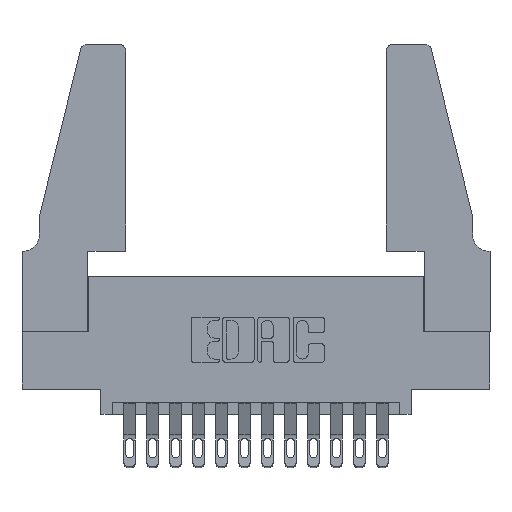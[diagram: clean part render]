
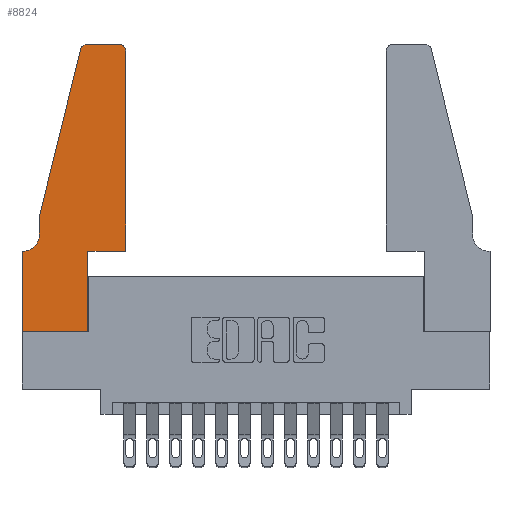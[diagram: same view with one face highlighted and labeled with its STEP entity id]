
A CAD part, top view. The second image highlights one B-rep face of the part: STEP entity #8824.
In plain terms, the highlighted planar face has unit normal (0, 0, 1).
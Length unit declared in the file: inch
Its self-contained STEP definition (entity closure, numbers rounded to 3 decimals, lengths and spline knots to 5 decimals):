
#144 = PLANE ( 'NONE',  #15446 ) ;
#333 = CARTESIAN_POINT ( 'NONE',  ( 0., 0.35, 0.37 ) ) ;
#470 = EDGE_CURVE ( 'NONE', #14573, #10132, #8382, .T. ) ;
#516 = ORIENTED_EDGE ( 'NONE', *, *, #2509, .T. ) ;
#527 = VECTOR ( 'NONE', #4725, 39.37008 ) ;
#585 = DIRECTION ( 'NONE',  ( 1., 0., 0. ) ) ;
#693 = CARTESIAN_POINT ( 'NONE',  ( 0.4205, 1.22, 0.37 ) ) ;
#936 = CARTESIAN_POINT ( 'NONE',  ( 0.0755, 0.35, 0.37 ) ) ;
#961 = EDGE_CURVE ( 'NONE', #8981, #6035, #6243, .T. ) ;
#1229 = ORIENTED_EDGE ( 'NONE', *, *, #961, .T. ) ;
#1365 = DIRECTION ( 'NONE',  ( 0., 0., 1. ) ) ;
#1646 = ORIENTED_EDGE ( 'NONE', *, *, #8129, .T. ) ;
#1683 = LINE ( 'NONE', #9833, #527 ) ;
#2045 = DIRECTION ( 'NONE',  ( 1., 0., 0. ) ) ;
#2175 = DIRECTION ( 'NONE',  ( -1., 0., 0. ) ) ;
#2217 = AXIS2_PLACEMENT_3D ( 'NONE', #10039, #11052, #11283 ) ;
#2308 = CARTESIAN_POINT ( 'NONE',  ( 0.4205, 1.25, 0.37 ) ) ;
#2393 = ORIENTED_EDGE ( 'NONE', *, *, #6255, .T. ) ;
#2509 = EDGE_CURVE ( 'NONE', #4810, #2697, #14955, .T. ) ;
#2515 = CIRCLE ( 'NONE', #7985, 0.03 ) ;
#2695 = ORIENTED_EDGE ( 'NONE', *, *, #9323, .T. ) ;
#2697 = VERTEX_POINT ( 'NONE', #333 ) ;
#2873 = EDGE_CURVE ( 'NONE', #10132, #11753, #2515, .T. ) ;
#3083 = CARTESIAN_POINT ( 'NONE',  ( 0.4505, 0.35, 0.37 ) ) ;
#3145 = VECTOR ( 'NONE', #15045, 39.37008 ) ;
#3296 = LINE ( 'NONE', #11211, #8168 ) ;
#3408 = VERTEX_POINT ( 'NONE', #14956 ) ;
#3936 = CARTESIAN_POINT ( 'NONE',  ( 0.2605, 1.25, 0.37 ) ) ;
#3981 = CARTESIAN_POINT ( 'NONE',  ( 0., 0., 0.37 ) ) ;
#4398 = AXIS2_PLACEMENT_3D ( 'NONE', #693, #10700, #10870 ) ;
#4725 = DIRECTION ( 'NONE',  ( -0.239, -0.971, 0. ) ) ;
#4736 = DIRECTION ( 'NONE',  ( 0., -1., 0. ) ) ;
#4810 = VERTEX_POINT ( 'NONE', #10640 ) ;
#5275 = VECTOR ( 'NONE', #4736, 39.37008 ) ;
#5314 = FACE_OUTER_BOUND ( 'NONE', #7008, .T. ) ;
#5336 = LINE ( 'NONE', #3083, #9787 ) ;
#5375 = VECTOR ( 'NONE', #15383, 39.37008 ) ;
#5434 = CARTESIAN_POINT ( 'NONE',  ( 0.25487, 1.22718, 0.37 ) ) ;
#5473 = VECTOR ( 'NONE', #14832, 39.37008 ) ;
#5708 = ORIENTED_EDGE ( 'NONE', *, *, #11734, .T. ) ;
#5768 = CARTESIAN_POINT ( 'NONE',  ( 0.0755, 0.5, 0.37 ) ) ;
#5809 = DIRECTION ( 'NONE',  ( 0., 1., 0. ) ) ;
#6035 = VERTEX_POINT ( 'NONE', #11112 ) ;
#6126 = ORIENTED_EDGE ( 'NONE', *, *, #14814, .T. ) ;
#6174 = CARTESIAN_POINT ( 'NONE',  ( 0.0755, 0.42, 0.37 ) ) ;
#6243 = LINE ( 'NONE', #7427, #5473 ) ;
#6255 = EDGE_CURVE ( 'NONE', #6035, #11138, #5336, .T. ) ;
#6564 = CIRCLE ( 'NONE', #2217, 0.07 ) ;
#6594 = LINE ( 'NONE', #11746, #13993 ) ;
#7008 = EDGE_LOOP ( 'NONE', ( #10977, #8465, #11889, #1646, #9849, #516, #6126, #14372, #5708, #1229, #2393, #2695 ) ) ;
#7026 = CARTESIAN_POINT ( 'NONE',  ( 0.284, 1.22, 0.37 ) ) ;
#7427 = CARTESIAN_POINT ( 'NONE',  ( 0.4505, 0.35, 0.37 ) ) ;
#7888 = LINE ( 'NONE', #11612, #5375 ) ;
#7943 = VERTEX_POINT ( 'NONE', #6174 ) ;
#7985 = AXIS2_PLACEMENT_3D ( 'NONE', #7026, #8079, #2045 ) ;
#8079 = DIRECTION ( 'NONE',  ( 0., 0., 1. ) ) ;
#8129 = EDGE_CURVE ( 'NONE', #11877, #7943, #14393, .T. ) ;
#8168 = VECTOR ( 'NONE', #11268, 39.37008 ) ;
#8382 = LINE ( 'NONE', #3936, #3145 ) ;
#8465 = ORIENTED_EDGE ( 'NONE', *, *, #2873, .T. ) ;
#8824 = ADVANCED_FACE ( 'NONE', ( #5314 ), #144, .T. ) ;
#8981 = VERTEX_POINT ( 'NONE', #11345 ) ;
#9234 = EDGE_CURVE ( 'NONE', #13243, #3408, #6594, .T. ) ;
#9323 = EDGE_CURVE ( 'NONE', #11138, #14573, #11806, .T. ) ;
#9787 = VECTOR ( 'NONE', #5809, 39.37008 ) ;
#9833 = CARTESIAN_POINT ( 'NONE',  ( 0.0755, 0.5, 0.37 ) ) ;
#9849 = ORIENTED_EDGE ( 'NONE', *, *, #10097, .T. ) ;
#10039 = CARTESIAN_POINT ( 'NONE',  ( 0.0055, 0.42, 0.37 ) ) ;
#10097 = EDGE_CURVE ( 'NONE', #7943, #4810, #6564, .T. ) ;
#10132 = VERTEX_POINT ( 'NONE', #12526 ) ;
#10640 = CARTESIAN_POINT ( 'NONE',  ( 0.0055, 0.35, 0.37 ) ) ;
#10700 = DIRECTION ( 'NONE',  ( 0., 0., 1. ) ) ;
#10870 = DIRECTION ( 'NONE',  ( 1., 0., 0. ) ) ;
#10912 = CARTESIAN_POINT ( 'NONE',  ( 0.0755, 0.5, 0.37 ) ) ;
#10977 = ORIENTED_EDGE ( 'NONE', *, *, #470, .T. ) ;
#11052 = DIRECTION ( 'NONE',  ( 0., 0., -1. ) ) ;
#11112 = CARTESIAN_POINT ( 'NONE',  ( 0.4505, 0.35, 0.37 ) ) ;
#11138 = VERTEX_POINT ( 'NONE', #14391 ) ;
#11206 = CARTESIAN_POINT ( 'NONE',  ( 0., 0.35, 0.37 ) ) ;
#11211 = CARTESIAN_POINT ( 'NONE',  ( 0., 0., 0.37 ) ) ;
#11268 = DIRECTION ( 'NONE',  ( 0., -1., 0. ) ) ;
#11283 = DIRECTION ( 'NONE',  ( -1., 0., 0. ) ) ;
#11345 = CARTESIAN_POINT ( 'NONE',  ( 0.2865, 0.35, 0.37 ) ) ;
#11506 = EDGE_CURVE ( 'NONE', #11753, #11877, #1683, .T. ) ;
#11612 = CARTESIAN_POINT ( 'NONE',  ( 0.2865, 0.35, 0.37 ) ) ;
#11734 = EDGE_CURVE ( 'NONE', #3408, #8981, #7888, .T. ) ;
#11746 = CARTESIAN_POINT ( 'NONE',  ( 0., 0., 0.37 ) ) ;
#11753 = VERTEX_POINT ( 'NONE', #5434 ) ;
#11806 = CIRCLE ( 'NONE', #4398, 0.03 ) ;
#11877 = VERTEX_POINT ( 'NONE', #5768 ) ;
#11889 = ORIENTED_EDGE ( 'NONE', *, *, #11506, .T. ) ;
#12526 = CARTESIAN_POINT ( 'NONE',  ( 0.284, 1.25, 0.37 ) ) ;
#13243 = VERTEX_POINT ( 'NONE', #3981 ) ;
#13785 = VECTOR ( 'NONE', #2175, 39.37008 ) ;
#13993 = VECTOR ( 'NONE', #585, 39.37008 ) ;
#14372 = ORIENTED_EDGE ( 'NONE', *, *, #9234, .T. ) ;
#14391 = CARTESIAN_POINT ( 'NONE',  ( 0.4505, 1.22, 0.37 ) ) ;
#14393 = LINE ( 'NONE', #10912, #5275 ) ;
#14573 = VERTEX_POINT ( 'NONE', #2308 ) ;
#14814 = EDGE_CURVE ( 'NONE', #2697, #13243, #3296, .T. ) ;
#14832 = DIRECTION ( 'NONE',  ( 1., 0., 0. ) ) ;
#14955 = LINE ( 'NONE', #936, #13785 ) ;
#14956 = CARTESIAN_POINT ( 'NONE',  ( 0.2865, 0., 0.37 ) ) ;
#14971 = DIRECTION ( 'NONE',  ( 1., 0., 0. ) ) ;
#15045 = DIRECTION ( 'NONE',  ( -1., 0., 0. ) ) ;
#15383 = DIRECTION ( 'NONE',  ( 0., 1., 0. ) ) ;
#15446 = AXIS2_PLACEMENT_3D ( 'NONE', #11206, #1365, #14971 ) ;
